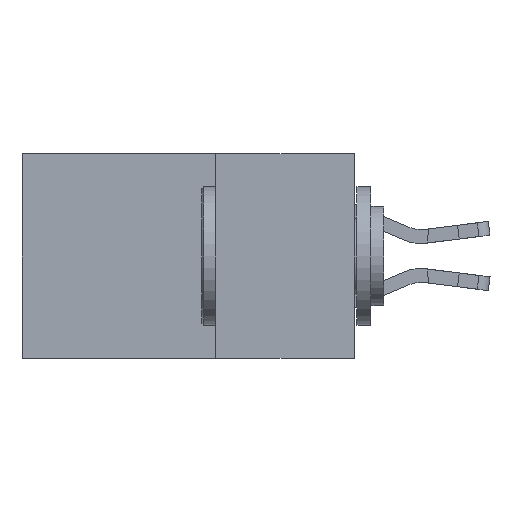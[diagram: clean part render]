
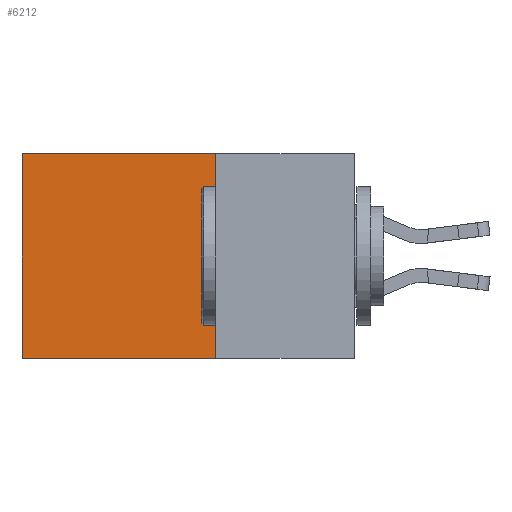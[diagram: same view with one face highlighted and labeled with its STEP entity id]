
A CAD part, left-side view. The second image highlights one B-rep face of the part: STEP entity #6212.
In plain terms, the highlighted planar face has unit normal (-1, 0, 0).
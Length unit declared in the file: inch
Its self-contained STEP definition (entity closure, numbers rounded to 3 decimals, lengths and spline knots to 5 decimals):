
#145 = PLANE ( 'NONE',  #1867 ) ;
#549 = VERTEX_POINT ( 'NONE', #7925 ) ;
#559 = ORIENTED_EDGE ( 'NONE', *, *, #6315, .F. ) ;
#894 = EDGE_LOOP ( 'NONE', ( #7545, #559, #3024, #5446 ) ) ;
#1344 = VERTEX_POINT ( 'NONE', #8879 ) ;
#1429 = LINE ( 'NONE', #10870, #3627 ) ;
#1482 = DIRECTION ( 'NONE',  ( 0., 0., -1. ) ) ;
#1867 = AXIS2_PLACEMENT_3D ( 'NONE', #6603, #7481, #2001 ) ;
#2001 = DIRECTION ( 'NONE',  ( 0., 0., -1. ) ) ;
#2745 = CARTESIAN_POINT ( 'NONE',  ( 0.2615, 0.6, 0. ) ) ;
#3024 = ORIENTED_EDGE ( 'NONE', *, *, #7104, .F. ) ;
#3114 = CARTESIAN_POINT ( 'NONE',  ( 0.2615, 0.25, -0.37 ) ) ;
#3346 = CARTESIAN_POINT ( 'NONE',  ( 0.2615, 0.6, -0.37 ) ) ;
#3466 = LINE ( 'NONE', #11021, #8227 ) ;
#3627 = VECTOR ( 'NONE', #6601, 39.37008 ) ;
#4631 = EDGE_CURVE ( 'NONE', #5464, #7536, #1429, .T. ) ;
#4897 = VECTOR ( 'NONE', #9342, 39.37008 ) ;
#5161 = FACE_OUTER_BOUND ( 'NONE', #894, .T. ) ;
#5446 = ORIENTED_EDGE ( 'NONE', *, *, #4631, .T. ) ;
#5464 = VERTEX_POINT ( 'NONE', #7907 ) ;
#5841 = DIRECTION ( 'NONE',  ( 0., 1., 0. ) ) ;
#6212 = ADVANCED_FACE ( 'NONE', ( #5161 ), #145, .F. ) ;
#6315 = EDGE_CURVE ( 'NONE', #549, #1344, #3466, .T. ) ;
#6601 = DIRECTION ( 'NONE',  ( 0., 1., 0. ) ) ;
#6603 = CARTESIAN_POINT ( 'NONE',  ( 0.2615, 0.25, -0.37 ) ) ;
#7104 = EDGE_CURVE ( 'NONE', #5464, #549, #9323, .T. ) ;
#7481 = DIRECTION ( 'NONE',  ( 1., 0., 0. ) ) ;
#7536 = VERTEX_POINT ( 'NONE', #2745 ) ;
#7545 = ORIENTED_EDGE ( 'NONE', *, *, #11134, .T. ) ;
#7907 = CARTESIAN_POINT ( 'NONE',  ( 0.2615, 0.25, 0. ) ) ;
#7925 = CARTESIAN_POINT ( 'NONE',  ( 0.2615, 0.25, -0.37 ) ) ;
#8227 = VECTOR ( 'NONE', #5841, 39.37008 ) ;
#8879 = CARTESIAN_POINT ( 'NONE',  ( 0.2615, 0.6, -0.37 ) ) ;
#9323 = LINE ( 'NONE', #3114, #4897 ) ;
#9342 = DIRECTION ( 'NONE',  ( 0., 0., -1. ) ) ;
#9902 = VECTOR ( 'NONE', #1482, 39.37008 ) ;
#10704 = LINE ( 'NONE', #3346, #9902 ) ;
#10870 = CARTESIAN_POINT ( 'NONE',  ( 0.2615, 0.25, 0. ) ) ;
#11021 = CARTESIAN_POINT ( 'NONE',  ( 0.2615, 0.25, -0.37 ) ) ;
#11134 = EDGE_CURVE ( 'NONE', #7536, #1344, #10704, .T. ) ;
